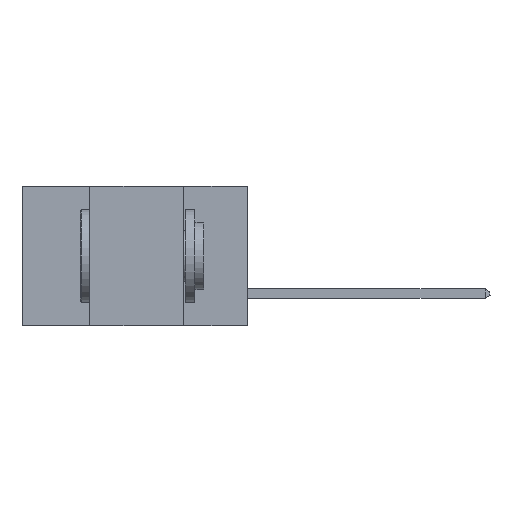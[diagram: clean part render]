
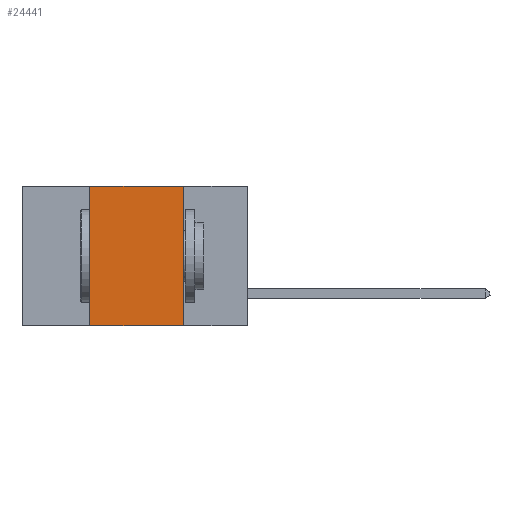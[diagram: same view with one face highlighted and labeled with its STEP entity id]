
A CAD part, left-side view. The second image highlights one B-rep face of the part: STEP entity #24441.
In plain terms, the highlighted planar face has unit normal (-1, 0, 0).
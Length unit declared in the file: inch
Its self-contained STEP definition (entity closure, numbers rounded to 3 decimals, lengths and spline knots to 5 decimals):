
#11 = VECTOR ( 'NONE', #10381, 39.37008 ) ;
#2001 = VERTEX_POINT ( 'NONE', #10126 ) ;
#2103 = LINE ( 'NONE', #6046, #12742 ) ;
#2238 = EDGE_LOOP ( 'NONE', ( #6878, #10324, #15045, #3469 ) ) ;
#3469 = ORIENTED_EDGE ( 'NONE', *, *, #12206, .T. ) ;
#4229 = DIRECTION ( 'NONE',  ( 0., 0., -1. ) ) ;
#5009 = DIRECTION ( 'NONE',  ( 0., -1., 0. ) ) ;
#5902 = VECTOR ( 'NONE', #5009, 39.37008 ) ;
#6046 = CARTESIAN_POINT ( 'NONE',  ( 0., 0.42, 0. ) ) ;
#6878 = ORIENTED_EDGE ( 'NONE', *, *, #18576, .F. ) ;
#7119 = VERTEX_POINT ( 'NONE', #20904 ) ;
#7378 = EDGE_CURVE ( 'NONE', #15569, #17024, #2103, .T. ) ;
#8694 = AXIS2_PLACEMENT_3D ( 'NONE', #15501, #27167, #4229 ) ;
#8864 = DIRECTION ( 'NONE',  ( 0., -1., 0. ) ) ;
#10126 = CARTESIAN_POINT ( 'NONE',  ( 0., 0.17, -0.37 ) ) ;
#10324 = ORIENTED_EDGE ( 'NONE', *, *, #13094, .F. ) ;
#10381 = DIRECTION ( 'NONE',  ( 0., 0., -1. ) ) ;
#12206 = EDGE_CURVE ( 'NONE', #15569, #2001, #19395, .T. ) ;
#12512 = CARTESIAN_POINT ( 'NONE',  ( 0., 0.6, 0. ) ) ;
#12519 = VECTOR ( 'NONE', #8864, 39.37008 ) ;
#12742 = VECTOR ( 'NONE', #21879, 39.37008 ) ;
#13094 = EDGE_CURVE ( 'NONE', #17024, #7119, #16116, .T. ) ;
#15045 = ORIENTED_EDGE ( 'NONE', *, *, #7378, .F. ) ;
#15397 = PLANE ( 'NONE',  #8694 ) ;
#15501 = CARTESIAN_POINT ( 'NONE',  ( 0., 0.6, 0. ) ) ;
#15569 = VERTEX_POINT ( 'NONE', #26443 ) ;
#16116 = LINE ( 'NONE', #12512, #12519 ) ;
#16723 = LINE ( 'NONE', #26076, #11 ) ;
#17024 = VERTEX_POINT ( 'NONE', #29163 ) ;
#18576 = EDGE_CURVE ( 'NONE', #7119, #2001, #16723, .T. ) ;
#19395 = LINE ( 'NONE', #22019, #5902 ) ;
#20904 = CARTESIAN_POINT ( 'NONE',  ( 0., 0.17, 0. ) ) ;
#21879 = DIRECTION ( 'NONE',  ( 0., 0., 1. ) ) ;
#22019 = CARTESIAN_POINT ( 'NONE',  ( 0., 0.6, -0.37 ) ) ;
#24441 = ADVANCED_FACE ( 'NONE', ( #28997 ), #15397, .F. ) ;
#26076 = CARTESIAN_POINT ( 'NONE',  ( 0., 0.17, 0. ) ) ;
#26443 = CARTESIAN_POINT ( 'NONE',  ( 0., 0.42, -0.37 ) ) ;
#27167 = DIRECTION ( 'NONE',  ( 1., 0., 0. ) ) ;
#28997 = FACE_OUTER_BOUND ( 'NONE', #2238, .T. ) ;
#29163 = CARTESIAN_POINT ( 'NONE',  ( 0., 0.42, 0. ) ) ;
